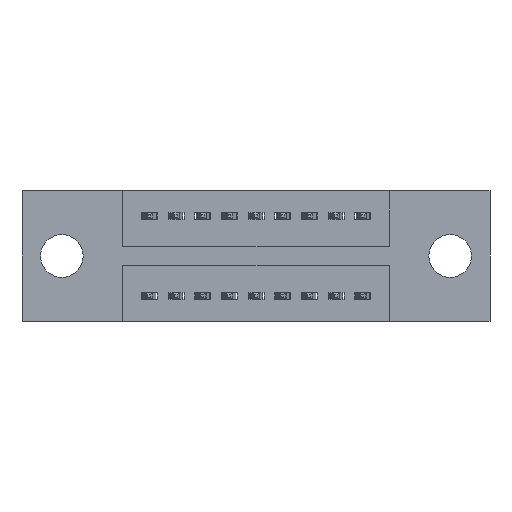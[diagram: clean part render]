
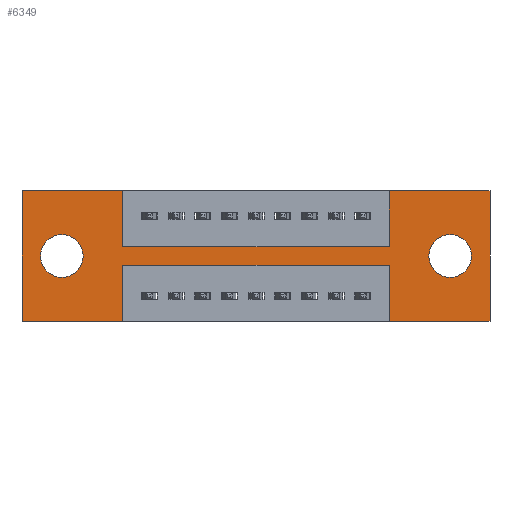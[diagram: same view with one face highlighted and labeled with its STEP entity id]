
A CAD part, front view. The second image highlights one B-rep face of the part: STEP entity #6349.
In plain terms, the highlighted planar face has unit normal (0, -1, 0).
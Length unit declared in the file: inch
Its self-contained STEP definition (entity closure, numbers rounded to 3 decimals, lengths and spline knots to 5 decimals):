
#131 = AXIS2_PLACEMENT_3D ( 'NONE', #1417, #5312, #7515 ) ;
#134 = EDGE_CURVE ( 'NONE', #3036, #6250, #3933, .T. ) ;
#215 = EDGE_CURVE ( 'NONE', #8444, #3925, #285, .T. ) ;
#285 = LINE ( 'NONE', #6337, #4790 ) ;
#377 = VECTOR ( 'NONE', #5291, 39.37008 ) ;
#399 = CARTESIAN_POINT ( 'NONE',  ( 1.3775, 0., -0.49 ) ) ;
#436 = VERTEX_POINT ( 'NONE', #6910 ) ;
#456 = ORIENTED_EDGE ( 'NONE', *, *, #4368, .F. ) ;
#508 = CARTESIAN_POINT ( 'NONE',  ( 0.1495, 0., -0.165 ) ) ;
#610 = VECTOR ( 'NONE', #6158, 39.37008 ) ;
#612 = DIRECTION ( 'NONE',  ( 0., 0., 1. ) ) ;
#743 = CARTESIAN_POINT ( 'NONE',  ( 0.3775, 0., -0.21 ) ) ;
#747 = CARTESIAN_POINT ( 'NONE',  ( 1.3775, 0., -0.21 ) ) ;
#760 = CARTESIAN_POINT ( 'NONE',  ( 0., 0., -0.49 ) ) ;
#763 = EDGE_CURVE ( 'NONE', #2068, #8053, #3683, .T. ) ;
#834 = AXIS2_PLACEMENT_3D ( 'NONE', #9304, #3944, #8770 ) ;
#977 = DIRECTION ( 'NONE',  ( 0., 1., 0. ) ) ;
#1092 = ORIENTED_EDGE ( 'NONE', *, *, #134, .F. ) ;
#1344 = CARTESIAN_POINT ( 'NONE',  ( 1.6055, 0., -0.245 ) ) ;
#1369 = EDGE_LOOP ( 'NONE', ( #7594, #4796 ) ) ;
#1409 = DIRECTION ( 'NONE',  ( 0., 0., -1. ) ) ;
#1417 = CARTESIAN_POINT ( 'NONE',  ( 0.1495, 0., -0.245 ) ) ;
#1513 = DIRECTION ( 'NONE',  ( 0., 0., -1. ) ) ;
#1545 = PLANE ( 'NONE',  #834 ) ;
#1606 = CARTESIAN_POINT ( 'NONE',  ( 0., 0., -0.49 ) ) ;
#1661 = DIRECTION ( 'NONE',  ( -1., 0., 0. ) ) ;
#1881 = DIRECTION ( 'NONE',  ( 0., 0., 1. ) ) ;
#2002 = EDGE_CURVE ( 'NONE', #5408, #7000, #4393, .T. ) ;
#2068 = VERTEX_POINT ( 'NONE', #4555 ) ;
#2206 = AXIS2_PLACEMENT_3D ( 'NONE', #1344, #3714, #1409 ) ;
#2225 = CARTESIAN_POINT ( 'NONE',  ( 1.755, 0., 0. ) ) ;
#2237 = EDGE_CURVE ( 'NONE', #8053, #6424, #4155, .T. ) ;
#2272 = LINE ( 'NONE', #7074, #8599 ) ;
#2297 = VERTEX_POINT ( 'NONE', #7044 ) ;
#2358 = CARTESIAN_POINT ( 'NONE',  ( 0., 0., 0. ) ) ;
#2442 = LINE ( 'NONE', #3450, #377 ) ;
#2445 = CARTESIAN_POINT ( 'NONE',  ( 1.3775, 0., -0.21 ) ) ;
#2563 = FACE_OUTER_BOUND ( 'NONE', #8228, .T. ) ;
#2610 = VECTOR ( 'NONE', #9538, 39.37008 ) ;
#2641 = LINE ( 'NONE', #7510, #5294 ) ;
#2715 = VECTOR ( 'NONE', #6413, 39.37008 ) ;
#2877 = EDGE_CURVE ( 'NONE', #3156, #3347, #7747, .T. ) ;
#2918 = FACE_BOUND ( 'NONE', #5043, .T. ) ;
#2971 = DIRECTION ( 'NONE',  ( 0., 1., 0. ) ) ;
#3001 = EDGE_CURVE ( 'NONE', #7000, #5408, #10019, .T. ) ;
#3026 = VECTOR ( 'NONE', #4428, 39.37008 ) ;
#3028 = CARTESIAN_POINT ( 'NONE',  ( 0., 0., 0. ) ) ;
#3036 = VERTEX_POINT ( 'NONE', #747 ) ;
#3103 = ORIENTED_EDGE ( 'NONE', *, *, #7167, .F. ) ;
#3156 = VERTEX_POINT ( 'NONE', #3345 ) ;
#3222 = DIRECTION ( 'NONE',  ( 0., 0., -1. ) ) ;
#3287 = ORIENTED_EDGE ( 'NONE', *, *, #7232, .F. ) ;
#3345 = CARTESIAN_POINT ( 'NONE',  ( 0.1495, 0., -0.325 ) ) ;
#3347 = VERTEX_POINT ( 'NONE', #508 ) ;
#3434 = VECTOR ( 'NONE', #8019, 39.37008 ) ;
#3450 = CARTESIAN_POINT ( 'NONE',  ( 0., 0., 0. ) ) ;
#3510 = ORIENTED_EDGE ( 'NONE', *, *, #2237, .F. ) ;
#3588 = VERTEX_POINT ( 'NONE', #399 ) ;
#3683 = LINE ( 'NONE', #1606, #2715 ) ;
#3714 = DIRECTION ( 'NONE',  ( 0., 1., 0. ) ) ;
#3883 = FACE_BOUND ( 'NONE', #1369, .T. ) ;
#3925 = VERTEX_POINT ( 'NONE', #7736 ) ;
#3933 = LINE ( 'NONE', #2445, #2610 ) ;
#3944 = DIRECTION ( 'NONE',  ( 0., -1., 0. ) ) ;
#4027 = LINE ( 'NONE', #5718, #3434 ) ;
#4097 = ORIENTED_EDGE ( 'NONE', *, *, #4710, .F. ) ;
#4155 = LINE ( 'NONE', #2358, #610 ) ;
#4343 = CARTESIAN_POINT ( 'NONE',  ( 0., 0., 0. ) ) ;
#4368 = EDGE_CURVE ( 'NONE', #6424, #436, #8727, .T. ) ;
#4393 = CIRCLE ( 'NONE', #6162, 0.08 ) ;
#4428 = DIRECTION ( 'NONE',  ( 0., 0., -1. ) ) ;
#4429 = ORIENTED_EDGE ( 'NONE', *, *, #5982, .F. ) ;
#4555 = CARTESIAN_POINT ( 'NONE',  ( 0.3775, 0., -0.49 ) ) ;
#4600 = ORIENTED_EDGE ( 'NONE', *, *, #5404, .F. ) ;
#4710 = EDGE_CURVE ( 'NONE', #7979, #2297, #2272, .T. ) ;
#4790 = VECTOR ( 'NONE', #1661, 39.37008 ) ;
#4796 = ORIENTED_EDGE ( 'NONE', *, *, #2877, .T. ) ;
#4929 = ORIENTED_EDGE ( 'NONE', *, *, #215, .F. ) ;
#5043 = EDGE_LOOP ( 'NONE', ( #8252, #7755 ) ) ;
#5199 = CARTESIAN_POINT ( 'NONE',  ( 1.6055, 0., -0.165 ) ) ;
#5291 = DIRECTION ( 'NONE',  ( 1., 0., 0. ) ) ;
#5294 = VECTOR ( 'NONE', #9111, 39.37008 ) ;
#5312 = DIRECTION ( 'NONE',  ( 0., 1., 0. ) ) ;
#5404 = EDGE_CURVE ( 'NONE', #3588, #8444, #5574, .T. ) ;
#5408 = VERTEX_POINT ( 'NONE', #5199 ) ;
#5574 = LINE ( 'NONE', #5916, #10068 ) ;
#5616 = EDGE_CURVE ( 'NONE', #3347, #3156, #7848, .T. ) ;
#5635 = CARTESIAN_POINT ( 'NONE',  ( 0.1495, 0., -0.245 ) ) ;
#5718 = CARTESIAN_POINT ( 'NONE',  ( 0.3775, 0., -0.21 ) ) ;
#5916 = CARTESIAN_POINT ( 'NONE',  ( 1.3775, 0., -0.28 ) ) ;
#5982 = EDGE_CURVE ( 'NONE', #7597, #3036, #4027, .T. ) ;
#6019 = DIRECTION ( 'NONE',  ( 0., 0., -1. ) ) ;
#6158 = DIRECTION ( 'NONE',  ( 0., 0., 1. ) ) ;
#6162 = AXIS2_PLACEMENT_3D ( 'NONE', #7562, #2971, #6019 ) ;
#6250 = VERTEX_POINT ( 'NONE', #9937 ) ;
#6337 = CARTESIAN_POINT ( 'NONE',  ( 0.3775, 0., -0.28 ) ) ;
#6349 = ADVANCED_FACE ( 'NONE', ( #2918, #3883, #2563 ), #1545, .T. ) ;
#6365 = AXIS2_PLACEMENT_3D ( 'NONE', #5635, #977, #1881 ) ;
#6413 = DIRECTION ( 'NONE',  ( -1., 0., 0. ) ) ;
#6424 = VERTEX_POINT ( 'NONE', #3028 ) ;
#6910 = CARTESIAN_POINT ( 'NONE',  ( 0.3775, 0., 0. ) ) ;
#7000 = VERTEX_POINT ( 'NONE', #8841 ) ;
#7044 = CARTESIAN_POINT ( 'NONE',  ( 1.755, 0., -0.49 ) ) ;
#7074 = CARTESIAN_POINT ( 'NONE',  ( 1.755, 0., 0. ) ) ;
#7167 = EDGE_CURVE ( 'NONE', #3925, #2068, #9465, .T. ) ;
#7232 = EDGE_CURVE ( 'NONE', #436, #7597, #7608, .T. ) ;
#7510 = CARTESIAN_POINT ( 'NONE',  ( 0., 0., -0.49 ) ) ;
#7515 = DIRECTION ( 'NONE',  ( 0., 0., 1. ) ) ;
#7562 = CARTESIAN_POINT ( 'NONE',  ( 1.6055, 0., -0.245 ) ) ;
#7594 = ORIENTED_EDGE ( 'NONE', *, *, #5616, .T. ) ;
#7597 = VERTEX_POINT ( 'NONE', #9223 ) ;
#7608 = LINE ( 'NONE', #743, #8109 ) ;
#7736 = CARTESIAN_POINT ( 'NONE',  ( 0.3775, 0., -0.28 ) ) ;
#7747 = CIRCLE ( 'NONE', #6365, 0.08 ) ;
#7755 = ORIENTED_EDGE ( 'NONE', *, *, #3001, .T. ) ;
#7848 = CIRCLE ( 'NONE', #131, 0.08 ) ;
#7855 = ORIENTED_EDGE ( 'NONE', *, *, #8486, .F. ) ;
#7979 = VERTEX_POINT ( 'NONE', #2225 ) ;
#8019 = DIRECTION ( 'NONE',  ( 1., 0., 0. ) ) ;
#8053 = VERTEX_POINT ( 'NONE', #760 ) ;
#8109 = VECTOR ( 'NONE', #1513, 39.37008 ) ;
#8228 = EDGE_LOOP ( 'NONE', ( #1092, #4429, #3287, #456, #3510, #9142, #3103, #4929, #4600, #7855, #4097, #8626 ) ) ;
#8252 = ORIENTED_EDGE ( 'NONE', *, *, #2002, .T. ) ;
#8444 = VERTEX_POINT ( 'NONE', #9002 ) ;
#8486 = EDGE_CURVE ( 'NONE', #2297, #3588, #2641, .T. ) ;
#8599 = VECTOR ( 'NONE', #3222, 39.37008 ) ;
#8626 = ORIENTED_EDGE ( 'NONE', *, *, #9268, .F. ) ;
#8727 = LINE ( 'NONE', #4343, #9215 ) ;
#8770 = DIRECTION ( 'NONE',  ( 0., 0., -1. ) ) ;
#8841 = CARTESIAN_POINT ( 'NONE',  ( 1.6055, 0., -0.325 ) ) ;
#9002 = CARTESIAN_POINT ( 'NONE',  ( 1.3775, 0., -0.28 ) ) ;
#9111 = DIRECTION ( 'NONE',  ( -1., 0., 0. ) ) ;
#9142 = ORIENTED_EDGE ( 'NONE', *, *, #763, .F. ) ;
#9165 = CARTESIAN_POINT ( 'NONE',  ( 0.3775, 0., -0.28 ) ) ;
#9215 = VECTOR ( 'NONE', #9726, 39.37008 ) ;
#9223 = CARTESIAN_POINT ( 'NONE',  ( 0.3775, 0., -0.21 ) ) ;
#9268 = EDGE_CURVE ( 'NONE', #6250, #7979, #2442, .T. ) ;
#9304 = CARTESIAN_POINT ( 'NONE',  ( 0., 0., -0.49 ) ) ;
#9465 = LINE ( 'NONE', #9165, #3026 ) ;
#9538 = DIRECTION ( 'NONE',  ( 0., 0., 1. ) ) ;
#9726 = DIRECTION ( 'NONE',  ( 1., 0., 0. ) ) ;
#9937 = CARTESIAN_POINT ( 'NONE',  ( 1.3775, 0., 0. ) ) ;
#10019 = CIRCLE ( 'NONE', #2206, 0.08 ) ;
#10068 = VECTOR ( 'NONE', #612, 39.37008 ) ;
